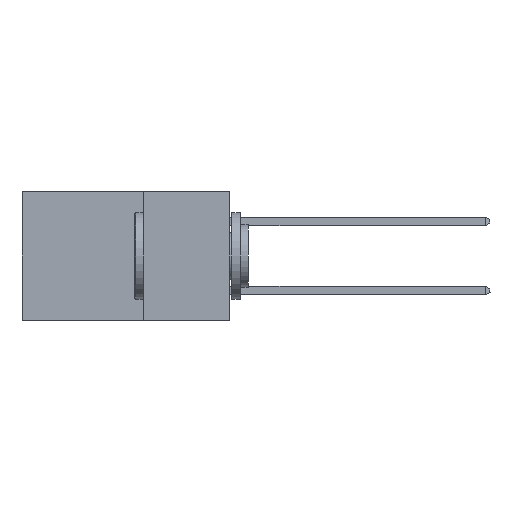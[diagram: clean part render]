
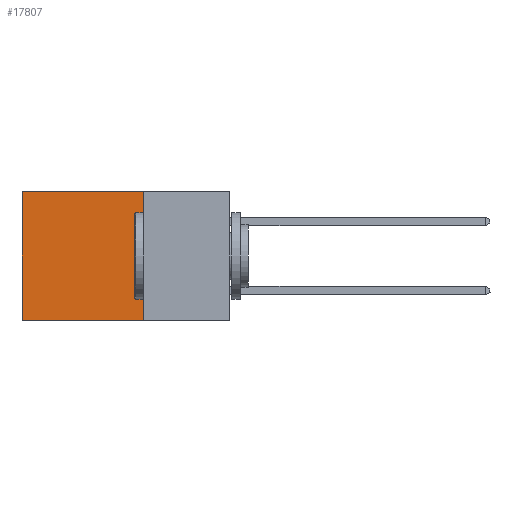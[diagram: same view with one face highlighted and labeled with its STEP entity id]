
A CAD part, left-side view. The second image highlights one B-rep face of the part: STEP entity #17807.
In plain terms, the highlighted planar face has unit normal (-1, 0, 0).
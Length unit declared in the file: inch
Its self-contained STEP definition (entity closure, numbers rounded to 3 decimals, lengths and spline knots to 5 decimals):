
#443 = DIRECTION ( 'NONE',  ( 1., 0., 0. ) ) ;
#1315 = ORIENTED_EDGE ( 'NONE', *, *, #6294, .T. ) ;
#1994 = DIRECTION ( 'NONE',  ( 0., 1., 0. ) ) ;
#2298 = AXIS2_PLACEMENT_3D ( 'NONE', #9393, #443, #18249 ) ;
#2669 = CARTESIAN_POINT ( 'NONE',  ( 0.298, 0.6, -0.37 ) ) ;
#4794 = CARTESIAN_POINT ( 'NONE',  ( 0.298, 0.6, 0. ) ) ;
#5227 = CARTESIAN_POINT ( 'NONE',  ( 0.298, 0.25, 0. ) ) ;
#5418 = VECTOR ( 'NONE', #1994, 39.37008 ) ;
#5903 = CARTESIAN_POINT ( 'NONE',  ( 0.298, 0.6, 0. ) ) ;
#6294 = EDGE_CURVE ( 'NONE', #10082, #15506, #13810, .T. ) ;
#7405 = CARTESIAN_POINT ( 'NONE',  ( 0.298, 0.25, -0.37 ) ) ;
#7537 = DIRECTION ( 'NONE',  ( 0., 0., -1. ) ) ;
#7844 = ORIENTED_EDGE ( 'NONE', *, *, #15041, .T. ) ;
#7907 = VECTOR ( 'NONE', #11373, 39.37008 ) ;
#8200 = VECTOR ( 'NONE', #16169, 39.37008 ) ;
#8425 = VERTEX_POINT ( 'NONE', #7405 ) ;
#8465 = ORIENTED_EDGE ( 'NONE', *, *, #15914, .F. ) ;
#8539 = EDGE_LOOP ( 'NONE', ( #7844, #9694, #8465, #1315 ) ) ;
#9052 = CARTESIAN_POINT ( 'NONE',  ( 0.298, 0.25, 0. ) ) ;
#9328 = PLANE ( 'NONE',  #2298 ) ;
#9393 = CARTESIAN_POINT ( 'NONE',  ( 0.298, 0.25, 0. ) ) ;
#9694 = ORIENTED_EDGE ( 'NONE', *, *, #16697, .F. ) ;
#10082 = VERTEX_POINT ( 'NONE', #9052 ) ;
#10619 = VECTOR ( 'NONE', #7537, 39.37008 ) ;
#11373 = DIRECTION ( 'NONE',  ( 0., 1., 0. ) ) ;
#12701 = LINE ( 'NONE', #13950, #5418 ) ;
#12873 = FACE_OUTER_BOUND ( 'NONE', #8539, .T. ) ;
#13810 = LINE ( 'NONE', #5227, #7907 ) ;
#13950 = CARTESIAN_POINT ( 'NONE',  ( 0.298, 0.25, -0.37 ) ) ;
#14786 = VERTEX_POINT ( 'NONE', #2669 ) ;
#14838 = LINE ( 'NONE', #5903, #10619 ) ;
#15041 = EDGE_CURVE ( 'NONE', #15506, #14786, #14838, .T. ) ;
#15506 = VERTEX_POINT ( 'NONE', #4794 ) ;
#15914 = EDGE_CURVE ( 'NONE', #10082, #8425, #18321, .T. ) ;
#16169 = DIRECTION ( 'NONE',  ( 0., 0., -1. ) ) ;
#16697 = EDGE_CURVE ( 'NONE', #8425, #14786, #12701, .T. ) ;
#17807 = ADVANCED_FACE ( 'NONE', ( #12873 ), #9328, .F. ) ;
#18249 = DIRECTION ( 'NONE',  ( 0., 0., -1. ) ) ;
#18321 = LINE ( 'NONE', #19459, #8200 ) ;
#19459 = CARTESIAN_POINT ( 'NONE',  ( 0.298, 0.25, 0. ) ) ;
